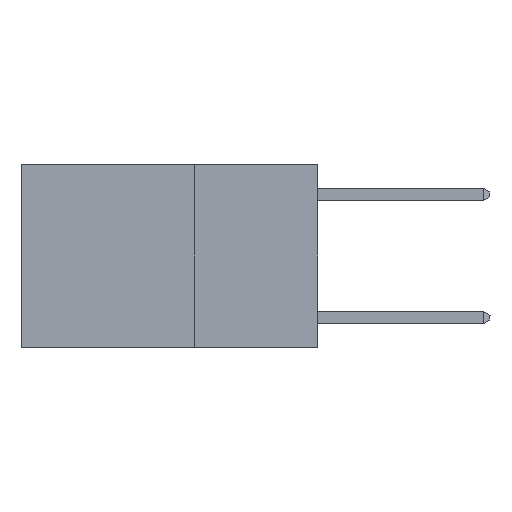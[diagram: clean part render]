
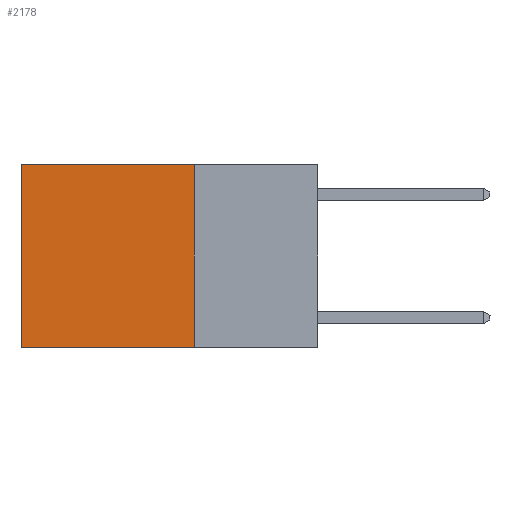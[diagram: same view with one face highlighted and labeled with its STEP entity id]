
A CAD part, left-side view. The second image highlights one B-rep face of the part: STEP entity #2178.
In plain terms, the highlighted planar face has unit normal (-1, 0, 0).
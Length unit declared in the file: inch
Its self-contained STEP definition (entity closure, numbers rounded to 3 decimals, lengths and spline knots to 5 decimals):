
#597 = DIRECTION ( 'NONE',  ( 1., 0., 0. ) ) ;
#751 = DIRECTION ( 'NONE',  ( 0., 1., 0. ) ) ;
#1072 = VERTEX_POINT ( 'NONE', #6574 ) ;
#1323 = CARTESIAN_POINT ( 'NONE',  ( 0.2625, 0.25, -0.37 ) ) ;
#1377 = CARTESIAN_POINT ( 'NONE',  ( 0.2625, 0.6, 0. ) ) ;
#1775 = DIRECTION ( 'NONE',  ( 0., 0., -1. ) ) ;
#1870 = PLANE ( 'NONE',  #8236 ) ;
#2178 = ADVANCED_FACE ( 'NONE', ( #6487 ), #1870, .F. ) ;
#2964 = CARTESIAN_POINT ( 'NONE',  ( 0.2625, 0.25, 0. ) ) ;
#3544 = EDGE_LOOP ( 'NONE', ( #9862, #7058, #12639, #7713 ) ) ;
#4596 = LINE ( 'NONE', #14083, #9204 ) ;
#5232 = VECTOR ( 'NONE', #751, 39.37008 ) ;
#5529 = EDGE_CURVE ( 'NONE', #6752, #1072, #13065, .T. ) ;
#6487 = FACE_OUTER_BOUND ( 'NONE', #3544, .T. ) ;
#6574 = CARTESIAN_POINT ( 'NONE',  ( 0.2625, 0.6, -0.37 ) ) ;
#6752 = VERTEX_POINT ( 'NONE', #7291 ) ;
#7058 = ORIENTED_EDGE ( 'NONE', *, *, #15050, .F. ) ;
#7063 = CARTESIAN_POINT ( 'NONE',  ( 0.2625, 0.25, 0. ) ) ;
#7090 = DIRECTION ( 'NONE',  ( 0., 1., 0. ) ) ;
#7291 = CARTESIAN_POINT ( 'NONE',  ( 0.2625, 0.6, 0. ) ) ;
#7713 = ORIENTED_EDGE ( 'NONE', *, *, #9761, .T. ) ;
#8236 = AXIS2_PLACEMENT_3D ( 'NONE', #2964, #597, #1775 ) ;
#8381 = CARTESIAN_POINT ( 'NONE',  ( 0.2625, 0.25, -0.37 ) ) ;
#8934 = LINE ( 'NONE', #8381, #14380 ) ;
#8991 = CARTESIAN_POINT ( 'NONE',  ( 0.2625, 0.25, 0. ) ) ;
#9204 = VECTOR ( 'NONE', #9433, 39.37008 ) ;
#9433 = DIRECTION ( 'NONE',  ( 0., 0., -1. ) ) ;
#9761 = EDGE_CURVE ( 'NONE', #12536, #6752, #14569, .T. ) ;
#9862 = ORIENTED_EDGE ( 'NONE', *, *, #5529, .T. ) ;
#11431 = VECTOR ( 'NONE', #13906, 39.37008 ) ;
#11674 = EDGE_CURVE ( 'NONE', #12536, #14572, #4596, .T. ) ;
#12536 = VERTEX_POINT ( 'NONE', #7063 ) ;
#12639 = ORIENTED_EDGE ( 'NONE', *, *, #11674, .F. ) ;
#13065 = LINE ( 'NONE', #1377, #11431 ) ;
#13906 = DIRECTION ( 'NONE',  ( 0., 0., -1. ) ) ;
#14083 = CARTESIAN_POINT ( 'NONE',  ( 0.2625, 0.25, 0. ) ) ;
#14380 = VECTOR ( 'NONE', #7090, 39.37008 ) ;
#14569 = LINE ( 'NONE', #8991, #5232 ) ;
#14572 = VERTEX_POINT ( 'NONE', #1323 ) ;
#15050 = EDGE_CURVE ( 'NONE', #14572, #1072, #8934, .T. ) ;
